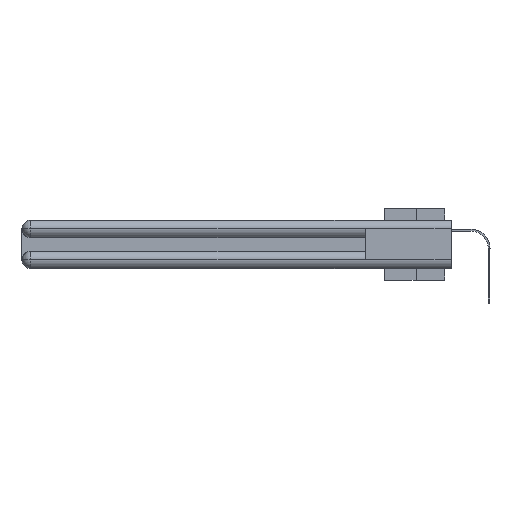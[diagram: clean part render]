
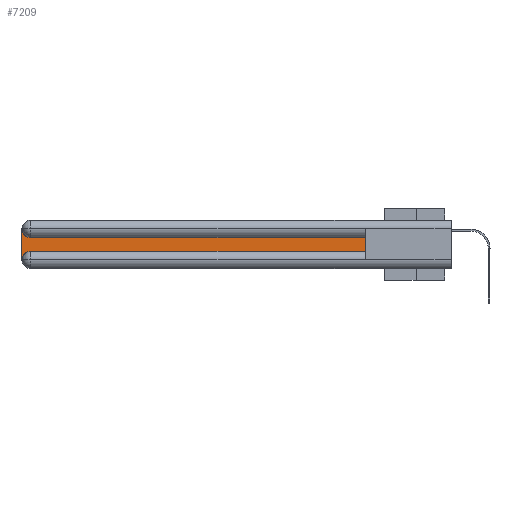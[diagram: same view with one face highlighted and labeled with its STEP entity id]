
A CAD part, left-side view. The second image highlights one B-rep face of the part: STEP entity #7209.
In plain terms, the highlighted planar face has unit normal (-1, 0, 0).
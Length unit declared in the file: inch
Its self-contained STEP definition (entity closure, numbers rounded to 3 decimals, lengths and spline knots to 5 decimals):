
#462 = LINE ( 'NONE', #37508, #32042 ) ;
#474 = LINE ( 'NONE', #6589, #25622 ) ;
#1740 = CIRCLE ( 'NONE', #34903, 0.06 ) ;
#1846 = CARTESIAN_POINT ( 'NONE',  ( 0.075, 2.94, -0.0625 ) ) ;
#2233 = ORIENTED_EDGE ( 'NONE', *, *, #38107, .T. ) ;
#2287 = CARTESIAN_POINT ( 'NONE',  ( 0.075, 0.6, -0.2175 ) ) ;
#2317 = CARTESIAN_POINT ( 'NONE',  ( 0.075, 0.6, -0.2175 ) ) ;
#4336 = EDGE_CURVE ( 'NONE', #37756, #22662, #462, .T. ) ;
#6394 = CARTESIAN_POINT ( 'NONE',  ( 0.075, 2.94, -0.1225 ) ) ;
#6589 = CARTESIAN_POINT ( 'NONE',  ( 0.075, 0.6, -0.1225 ) ) ;
#7209 = ADVANCED_FACE ( 'NONE', ( #27105 ), #11629, .F. ) ;
#7557 = ORIENTED_EDGE ( 'NONE', *, *, #25187, .T. ) ;
#7957 = CARTESIAN_POINT ( 'NONE',  ( 0.075, 3., -0.2175 ) ) ;
#9420 = VERTEX_POINT ( 'NONE', #6394 ) ;
#9508 = ORIENTED_EDGE ( 'NONE', *, *, #32055, .T. ) ;
#10161 = CARTESIAN_POINT ( 'NONE',  ( 0.075, 3., -0.0625 ) ) ;
#10589 = CARTESIAN_POINT ( 'NONE',  ( 0.075, 3., -0.2775 ) ) ;
#10736 = ORIENTED_EDGE ( 'NONE', *, *, #4336, .T. ) ;
#10885 = EDGE_CURVE ( 'NONE', #19164, #37756, #20194, .T. ) ;
#11629 = PLANE ( 'NONE',  #30753 ) ;
#14374 = DIRECTION ( 'NONE',  ( 1., 0., 0. ) ) ;
#16536 = DIRECTION ( 'NONE',  ( 0., 0., 1. ) ) ;
#17108 = DIRECTION ( 'NONE',  ( 1., 0., 0. ) ) ;
#17545 = CARTESIAN_POINT ( 'NONE',  ( 0.075, 3., -0.1225 ) ) ;
#18022 = CIRCLE ( 'NONE', #23206, 0.06 ) ;
#19045 = ORIENTED_EDGE ( 'NONE', *, *, #10885, .T. ) ;
#19164 = VERTEX_POINT ( 'NONE', #31120 ) ;
#19889 = CARTESIAN_POINT ( 'NONE',  ( 0.075, 2.94, -0.2775 ) ) ;
#20194 = LINE ( 'NONE', #2287, #36766 ) ;
#22662 = VERTEX_POINT ( 'NONE', #31788 ) ;
#23206 = AXIS2_PLACEMENT_3D ( 'NONE', #1846, #17108, #38077 ) ;
#23516 = DIRECTION ( 'NONE',  ( 0., 0., -1. ) ) ;
#24038 = DIRECTION ( 'NONE',  ( 0., 0., -1. ) ) ;
#25187 = EDGE_CURVE ( 'NONE', #22662, #9420, #474, .T. ) ;
#25622 = VECTOR ( 'NONE', #32364, 39.37008 ) ;
#27105 = FACE_OUTER_BOUND ( 'NONE', #35455, .T. ) ;
#28471 = EDGE_CURVE ( 'NONE', #9420, #29951, #18022, .T. ) ;
#29781 = DIRECTION ( 'NONE',  ( 0., -1., 0. ) ) ;
#29951 = VERTEX_POINT ( 'NONE', #10161 ) ;
#30753 = AXIS2_PLACEMENT_3D ( 'NONE', #17545, #35682, #24038 ) ;
#31120 = CARTESIAN_POINT ( 'NONE',  ( 0.075, 2.94, -0.2175 ) ) ;
#31788 = CARTESIAN_POINT ( 'NONE',  ( 0.075, 0.6, -0.1225 ) ) ;
#32042 = VECTOR ( 'NONE', #16536, 39.37008 ) ;
#32055 = EDGE_CURVE ( 'NONE', #37246, #19164, #1740, .T. ) ;
#32364 = DIRECTION ( 'NONE',  ( 0., 1., 0. ) ) ;
#32804 = LINE ( 'NONE', #7957, #39069 ) ;
#34903 = AXIS2_PLACEMENT_3D ( 'NONE', #19889, #14374, #23516 ) ;
#35250 = DIRECTION ( 'NONE',  ( 0., 0., -1. ) ) ;
#35455 = EDGE_LOOP ( 'NONE', ( #7557, #37355, #2233, #9508, #19045, #10736 ) ) ;
#35682 = DIRECTION ( 'NONE',  ( 1., 0., 0. ) ) ;
#36766 = VECTOR ( 'NONE', #29781, 39.37008 ) ;
#37246 = VERTEX_POINT ( 'NONE', #10589 ) ;
#37355 = ORIENTED_EDGE ( 'NONE', *, *, #28471, .T. ) ;
#37508 = CARTESIAN_POINT ( 'NONE',  ( 0.075, 0.6, -0.2175 ) ) ;
#37756 = VERTEX_POINT ( 'NONE', #2317 ) ;
#38077 = DIRECTION ( 'NONE',  ( 0., 0., -1. ) ) ;
#38107 = EDGE_CURVE ( 'NONE', #29951, #37246, #32804, .T. ) ;
#39069 = VECTOR ( 'NONE', #35250, 39.37008 ) ;
